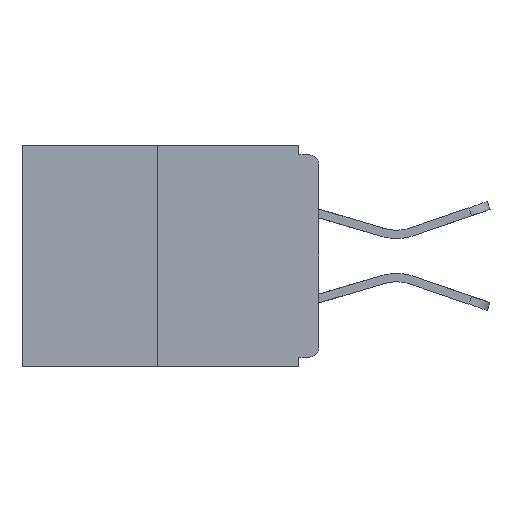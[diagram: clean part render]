
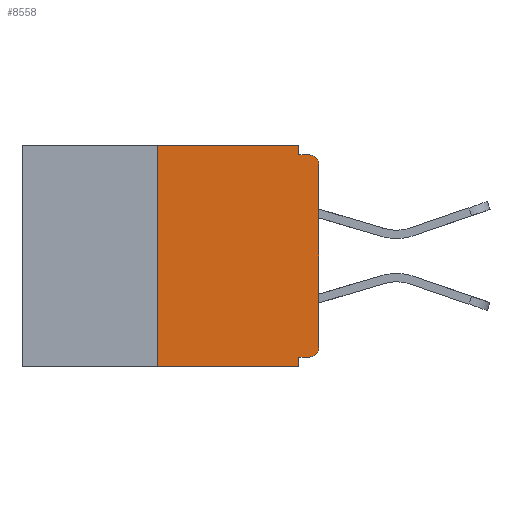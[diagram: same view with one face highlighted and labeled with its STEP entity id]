
A CAD part, left-side view. The second image highlights one B-rep face of the part: STEP entity #8558.
In plain terms, the highlighted planar face has unit normal (-1, 0, 0).
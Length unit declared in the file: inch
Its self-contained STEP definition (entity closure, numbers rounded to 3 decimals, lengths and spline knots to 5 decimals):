
#224 = DIRECTION ( 'NONE',  ( 0., 0., -1. ) ) ;
#671 = VERTEX_POINT ( 'NONE', #5685 ) ;
#981 = ORIENTED_EDGE ( 'NONE', *, *, #2801, .T. ) ;
#1586 = CARTESIAN_POINT ( 'NONE',  ( 0., 0.015, -0.015 ) ) ;
#2474 = CARTESIAN_POINT ( 'NONE',  ( 0., 0., -0.328 ) ) ;
#2546 = DIRECTION ( 'NONE',  ( 1., 0., 0. ) ) ;
#2685 = VERTEX_POINT ( 'NONE', #3558 ) ;
#2801 = EDGE_CURVE ( 'NONE', #2685, #8267, #6028, .T. ) ;
#3188 = ORIENTED_EDGE ( 'NONE', *, *, #13772, .T. ) ;
#3251 = ORIENTED_EDGE ( 'NONE', *, *, #20609, .F. ) ;
#3362 = VERTEX_POINT ( 'NONE', #22067 ) ;
#3558 = CARTESIAN_POINT ( 'NONE',  ( 0., 0., -0.03 ) ) ;
#3797 = CARTESIAN_POINT ( 'NONE',  ( 0., 0.031, -0.343 ) ) ;
#3967 = EDGE_CURVE ( 'NONE', #17590, #20732, #9911, .T. ) ;
#4854 = DIRECTION ( 'NONE',  ( 0., 0., 1. ) ) ;
#5146 = VECTOR ( 'NONE', #16271, 39.37008 ) ;
#5268 = LINE ( 'NONE', #13063, #13127 ) ;
#5527 = VECTOR ( 'NONE', #15972, 39.37008 ) ;
#5685 = CARTESIAN_POINT ( 'NONE',  ( 0., 0.031, 0. ) ) ;
#6028 = CIRCLE ( 'NONE', #19003, 0.015 ) ;
#6044 = ORIENTED_EDGE ( 'NONE', *, *, #3967, .F. ) ;
#6174 = VECTOR ( 'NONE', #16696, 39.37008 ) ;
#6310 = LINE ( 'NONE', #20033, #8006 ) ;
#6665 = VECTOR ( 'NONE', #21080, 39.37008 ) ;
#6792 = CARTESIAN_POINT ( 'NONE',  ( 0., 0.25, -0.343 ) ) ;
#7322 = VERTEX_POINT ( 'NONE', #3797 ) ;
#7432 = DIRECTION ( 'NONE',  ( 0., 0., -1. ) ) ;
#7759 = CIRCLE ( 'NONE', #22785, 0.015 ) ;
#7909 = EDGE_CURVE ( 'NONE', #671, #19518, #8066, .T. ) ;
#7979 = CARTESIAN_POINT ( 'NONE',  ( 0., 0., -0.313 ) ) ;
#8006 = VECTOR ( 'NONE', #224, 39.37008 ) ;
#8066 = LINE ( 'NONE', #10564, #5527 ) ;
#8085 = ORIENTED_EDGE ( 'NONE', *, *, #7909, .F. ) ;
#8267 = VERTEX_POINT ( 'NONE', #1586 ) ;
#8459 = ORIENTED_EDGE ( 'NONE', *, *, #23024, .F. ) ;
#8558 = ADVANCED_FACE ( 'NONE', ( #19114 ), #15567, .F. ) ;
#8881 = CARTESIAN_POINT ( 'NONE',  ( 0., 0.46, 0. ) ) ;
#9080 = EDGE_LOOP ( 'NONE', ( #8459, #6044, #13393, #12658, #20607, #3188, #10869, #981, #3251, #8085 ) ) ;
#9911 = LINE ( 'NONE', #20889, #18887 ) ;
#10339 = LINE ( 'NONE', #16099, #18749 ) ;
#10564 = CARTESIAN_POINT ( 'NONE',  ( 0., 0.031, 0. ) ) ;
#10869 = ORIENTED_EDGE ( 'NONE', *, *, #11784, .T. ) ;
#11171 = EDGE_CURVE ( 'NONE', #3362, #17324, #12896, .T. ) ;
#11253 = CARTESIAN_POINT ( 'NONE',  ( 0., 0.015, -0.03 ) ) ;
#11256 = DIRECTION ( 'NONE',  ( 0., 0., -1. ) ) ;
#11543 = CARTESIAN_POINT ( 'NONE',  ( 0., 0.25, 0. ) ) ;
#11784 = EDGE_CURVE ( 'NONE', #14283, #2685, #5268, .T. ) ;
#11971 = DIRECTION ( 'NONE',  ( 0., 0., 1. ) ) ;
#12077 = CARTESIAN_POINT ( 'NONE',  ( 0., 0.031, -0.015 ) ) ;
#12658 = ORIENTED_EDGE ( 'NONE', *, *, #13822, .F. ) ;
#12896 = LINE ( 'NONE', #2474, #6174 ) ;
#13063 = CARTESIAN_POINT ( 'NONE',  ( 0., 0., 0. ) ) ;
#13127 = VECTOR ( 'NONE', #11971, 39.37008 ) ;
#13393 = ORIENTED_EDGE ( 'NONE', *, *, #21953, .T. ) ;
#13772 = EDGE_CURVE ( 'NONE', #3362, #14283, #7759, .T. ) ;
#13822 = EDGE_CURVE ( 'NONE', #17324, #7322, #6310, .T. ) ;
#14283 = VERTEX_POINT ( 'NONE', #7979 ) ;
#14709 = LINE ( 'NONE', #16184, #5146 ) ;
#14828 = DIRECTION ( 'NONE',  ( -1., 0., 0. ) ) ;
#15567 = PLANE ( 'NONE',  #19386 ) ;
#15972 = DIRECTION ( 'NONE',  ( 0., 0., -1. ) ) ;
#16099 = CARTESIAN_POINT ( 'NONE',  ( 0., 0.46, -0.343 ) ) ;
#16184 = CARTESIAN_POINT ( 'NONE',  ( 0., 0., -0.015 ) ) ;
#16271 = DIRECTION ( 'NONE',  ( 0., -1., 0. ) ) ;
#16696 = DIRECTION ( 'NONE',  ( 0., 1., 0. ) ) ;
#17270 = DIRECTION ( 'NONE',  ( 0., 0., -1. ) ) ;
#17324 = VERTEX_POINT ( 'NONE', #18400 ) ;
#17590 = VERTEX_POINT ( 'NONE', #6792 ) ;
#18400 = CARTESIAN_POINT ( 'NONE',  ( 0., 0.031, -0.328 ) ) ;
#18749 = VECTOR ( 'NONE', #19633, 39.37008 ) ;
#18887 = VECTOR ( 'NONE', #4854, 39.37008 ) ;
#19003 = AXIS2_PLACEMENT_3D ( 'NONE', #11253, #14828, #7432 ) ;
#19114 = FACE_OUTER_BOUND ( 'NONE', #9080, .T. ) ;
#19386 = AXIS2_PLACEMENT_3D ( 'NONE', #21258, #2546, #17270 ) ;
#19518 = VERTEX_POINT ( 'NONE', #12077 ) ;
#19633 = DIRECTION ( 'NONE',  ( 0., -1., 0. ) ) ;
#20033 = CARTESIAN_POINT ( 'NONE',  ( 0., 0.031, -0.343 ) ) ;
#20182 = DIRECTION ( 'NONE',  ( -1., 0., 0. ) ) ;
#20607 = ORIENTED_EDGE ( 'NONE', *, *, #11171, .F. ) ;
#20609 = EDGE_CURVE ( 'NONE', #19518, #8267, #14709, .T. ) ;
#20689 = LINE ( 'NONE', #8881, #6665 ) ;
#20732 = VERTEX_POINT ( 'NONE', #11543 ) ;
#20889 = CARTESIAN_POINT ( 'NONE',  ( 0., 0.25, 0. ) ) ;
#21080 = DIRECTION ( 'NONE',  ( 0., -1., 0. ) ) ;
#21258 = CARTESIAN_POINT ( 'NONE',  ( 0., 0.46, 0. ) ) ;
#21846 = CARTESIAN_POINT ( 'NONE',  ( 0., 0.015, -0.313 ) ) ;
#21953 = EDGE_CURVE ( 'NONE', #17590, #7322, #10339, .T. ) ;
#22067 = CARTESIAN_POINT ( 'NONE',  ( 0., 0.015, -0.328 ) ) ;
#22785 = AXIS2_PLACEMENT_3D ( 'NONE', #21846, #20182, #11256 ) ;
#23024 = EDGE_CURVE ( 'NONE', #20732, #671, #20689, .T. ) ;
